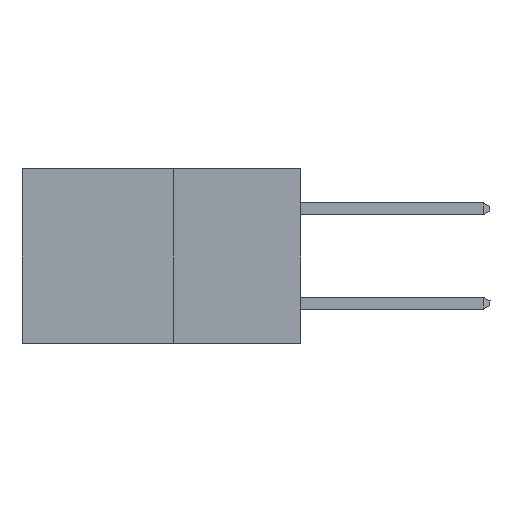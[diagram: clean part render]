
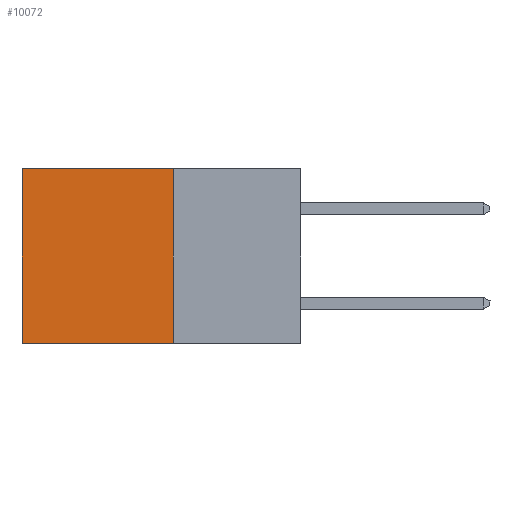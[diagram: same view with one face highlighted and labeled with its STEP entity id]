
A CAD part, left-side view. The second image highlights one B-rep face of the part: STEP entity #10072.
In plain terms, the highlighted planar face has unit normal (-1, 0, 0).
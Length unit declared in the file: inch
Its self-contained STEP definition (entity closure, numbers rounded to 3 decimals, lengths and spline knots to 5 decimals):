
#62 = VERTEX_POINT ( 'NONE', #5139 ) ;
#646 = CARTESIAN_POINT ( 'NONE',  ( 0.277, 0.59, -0.37 ) ) ;
#1337 = CARTESIAN_POINT ( 'NONE',  ( 0.277, 0.27, -0.37 ) ) ;
#1419 = EDGE_CURVE ( 'NONE', #62, #6673, #6477, .T. ) ;
#1564 = VECTOR ( 'NONE', #7559, 39.37008 ) ;
#2299 = DIRECTION ( 'NONE',  ( 0., 1., 0. ) ) ;
#2310 = ORIENTED_EDGE ( 'NONE', *, *, #1419, .F. ) ;
#2404 = ORIENTED_EDGE ( 'NONE', *, *, #9727, .T. ) ;
#2420 = DIRECTION ( 'NONE',  ( 0., 0., -1. ) ) ;
#2997 = CARTESIAN_POINT ( 'NONE',  ( 0.277, 0.27, -0.37 ) ) ;
#3583 = VECTOR ( 'NONE', #4624, 39.37008 ) ;
#4037 = ORIENTED_EDGE ( 'NONE', *, *, #10145, .T. ) ;
#4047 = ORIENTED_EDGE ( 'NONE', *, *, #8107, .F. ) ;
#4624 = DIRECTION ( 'NONE',  ( 0., 1., 0. ) ) ;
#4642 = DIRECTION ( 'NONE',  ( 0., 0., -1. ) ) ;
#5139 = CARTESIAN_POINT ( 'NONE',  ( 0.277, 0.27, 0. ) ) ;
#5852 = CARTESIAN_POINT ( 'NONE',  ( 0.277, 0.27, -0.37 ) ) ;
#6075 = LINE ( 'NONE', #8586, #3583 ) ;
#6477 = LINE ( 'NONE', #6884, #8319 ) ;
#6592 = VERTEX_POINT ( 'NONE', #9432 ) ;
#6660 = EDGE_LOOP ( 'NONE', ( #4037, #4047, #2310, #2404 ) ) ;
#6662 = PLANE ( 'NONE',  #9535 ) ;
#6673 = VERTEX_POINT ( 'NONE', #2997 ) ;
#6884 = CARTESIAN_POINT ( 'NONE',  ( 0.277, 0.27, -0.37 ) ) ;
#7452 = DIRECTION ( 'NONE',  ( 1., 0., 0. ) ) ;
#7559 = DIRECTION ( 'NONE',  ( 0., 0., -1. ) ) ;
#7697 = VERTEX_POINT ( 'NONE', #10878 ) ;
#8107 = EDGE_CURVE ( 'NONE', #6673, #6592, #10782, .T. ) ;
#8319 = VECTOR ( 'NONE', #4642, 39.37008 ) ;
#8573 = VECTOR ( 'NONE', #2299, 39.37008 ) ;
#8586 = CARTESIAN_POINT ( 'NONE',  ( 0.277, 0.27, 0. ) ) ;
#9057 = FACE_OUTER_BOUND ( 'NONE', #6660, .T. ) ;
#9432 = CARTESIAN_POINT ( 'NONE',  ( 0.277, 0.59, -0.37 ) ) ;
#9535 = AXIS2_PLACEMENT_3D ( 'NONE', #5852, #7452, #2420 ) ;
#9727 = EDGE_CURVE ( 'NONE', #62, #7697, #6075, .T. ) ;
#10072 = ADVANCED_FACE ( 'NONE', ( #9057 ), #6662, .F. ) ;
#10145 = EDGE_CURVE ( 'NONE', #7697, #6592, #10753, .T. ) ;
#10753 = LINE ( 'NONE', #646, #1564 ) ;
#10782 = LINE ( 'NONE', #1337, #8573 ) ;
#10878 = CARTESIAN_POINT ( 'NONE',  ( 0.277, 0.59, 0. ) ) ;
